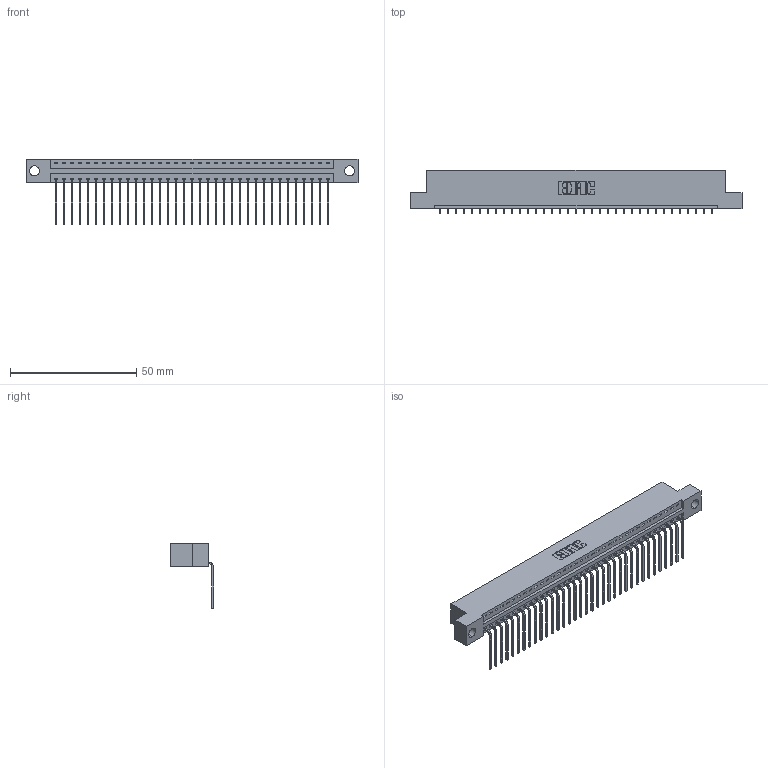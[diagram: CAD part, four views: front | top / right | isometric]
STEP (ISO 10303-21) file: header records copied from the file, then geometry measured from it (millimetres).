
FILE_DESCRIPTION (( 'STEP AP203' ), '1' );
FILE_NAME ('396-035-559-104.STEP', '2018-09-06T03:04:11', ( '' ), ( '' ), 'SwSTEP 2.0', 'SolidWorks 2016', '' );
FILE_SCHEMA (( 'CONFIG_CONTROL_DESIGN' ));
Length unit declared in the file: inch
Products named in the file (3): 345-292-001_558 559 Tail - 1; 396-035-559-104; 346 Part_Flush Mounting Lugs - 0.156 Dia-TH
Assembly tree (36 placements, depth 2):
  396-035-559-104
    346 Part_Flush Mounting Lugs - 0.156 Dia-TH
    345-292-001_558 559 Tail - 1  x35
Bounding box: 131.7 x 17.08 x 26.16 mm (x, y, z)
Volume: 12587 mm3; surface area: 16157.3 mm2
Topology: 36 solids, 36 shells, 2222 faces, 6699 edges, 4418 vertices
Faces by surface type: plane 1546, cylinder 676
Entity records: 22751 total; most frequent: CARTESIAN_POINT 3909, ORIENTED_EDGE 3878, DIRECTION 3457, EDGE_CURVE 1939, VECTOR 1667, LINE 1667, VERTEX_POINT 1290, AXIS2_PLACEMENT_3D 895
